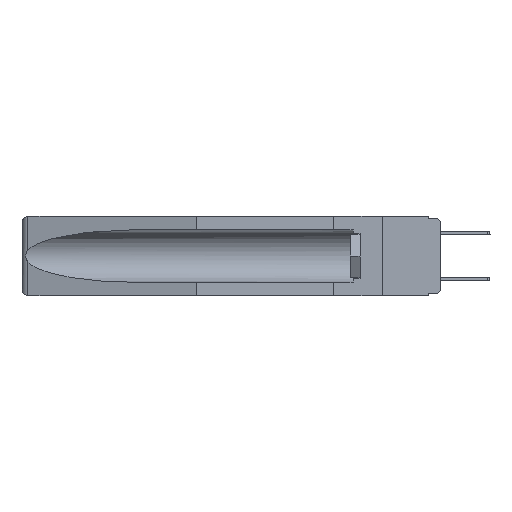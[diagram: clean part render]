
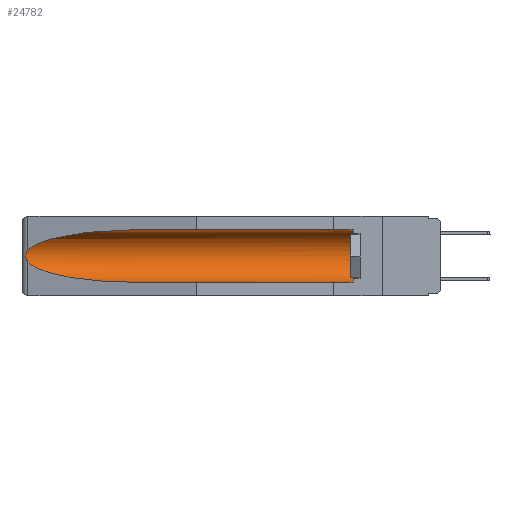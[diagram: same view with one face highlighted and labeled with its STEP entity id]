
A CAD part, left-side view. The second image highlights one B-rep face of the part: STEP entity #24782.
In plain terms, the highlighted cylindrical face has radius 2.857 mm (diameter 5.715 mm), a partial arc.
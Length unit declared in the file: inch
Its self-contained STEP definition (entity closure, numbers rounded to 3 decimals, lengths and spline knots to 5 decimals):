
#196 = DIRECTION ( 'NONE',  ( 0., 0., 1. ) ) ;
#798 = DIRECTION ( 'NONE',  ( 0., 1., 0. ) ) ;
#1414 = CARTESIAN_POINT ( 'NONE',  ( 0.2675, 1.53308, -0.17534 ) ) ;
#1496 = EDGE_CURVE ( 'NONE', #23119, #3552, #24272, .T. ) ;
#1505 = CARTESIAN_POINT ( 'NONE',  ( 0.2673, 1.5327, -0.16383 ) ) ;
#2046 = VERTEX_POINT ( 'NONE', #22098 ) ;
#2772 = CARTESIAN_POINT ( 'NONE',  ( 0.21114, 1.30732, -0.284 ) ) ;
#3189 = CARTESIAN_POINT ( 'NONE',  ( 0.155, 1.07973, -0.059 ) ) ;
#3433 = EDGE_CURVE ( 'NONE', #20549, #22015, #21277, .T. ) ;
#3552 = VERTEX_POINT ( 'NONE', #7488 ) ;
#4908 = ORIENTED_EDGE ( 'NONE', *, *, #1496, .T. ) ;
#5174 = EDGE_CURVE ( 'NONE', #2046, #26042, #6064, .T. ) ;
#5213 = EDGE_CURVE ( 'NONE', #20549, #23119, #16627, .T. ) ;
#6064 = B_SPLINE_CURVE_WITH_KNOTS ( 'NONE', 3,
 ( #16032, #22085, #18098, #1505, #9717, #1414, #24068, #21994, #17839, #19730 ),
 .UNSPECIFIED., .F., .F.,
 ( 4, 2, 2, 2, 4 ),
 ( 0., 0.00029, 0.00058, 0.00087, 0.00117 ),
 .UNSPECIFIED. ) ;
#6332 = EDGE_CURVE ( 'NONE', #26042, #22015, #12840, .T. ) ;
#6385 = CARTESIAN_POINT ( 'NONE',  ( 0.155, 0.126, -0.059 ) ) ;
#7488 = CARTESIAN_POINT ( 'NONE',  ( 0.155, 1.07973, -0.059 ) ) ;
#7738 = DIRECTION ( 'NONE',  ( 0., 0., 1. ) ) ;
#7851 = ORIENTED_EDGE ( 'NONE', *, *, #5174, .T. ) ;
#8418 = EDGE_LOOP ( 'NONE', ( #22985, #7851, #19996, #12005, #13705, #4908 ) ) ;
#8520 = CARTESIAN_POINT ( 'NONE',  ( 0.155, -0.30754, -0.284 ) ) ;
#9717 = CARTESIAN_POINT ( 'NONE',  ( 0.2675, 1.53308, -0.16763 ) ) ;
#10247 = CYLINDRICAL_SURFACE ( 'NONE', #12475, 0.1125 ) ;
#10984 = CARTESIAN_POINT ( 'NONE',  ( 0.25451, 1.48313, -0.24835 ) ) ;
#11436 = AXIS2_PLACEMENT_3D ( 'NONE', #20095, #11538, #7738 ) ;
#11538 = DIRECTION ( 'NONE',  ( 0., -1., 0. ) ) ;
#12005 = ORIENTED_EDGE ( 'NONE', *, *, #3433, .F. ) ;
#12475 = AXIS2_PLACEMENT_3D ( 'NONE', #20961, #12591, #196 ) ;
#12591 = DIRECTION ( 'NONE',  ( 0., 1., 0. ) ) ;
#12840 =( BOUNDED_CURVE ( )  B_SPLINE_CURVE ( 3, ( #14835, #10984, #2772, #13651 ),
 .UNSPECIFIED., .F., .T. ) 
 B_SPLINE_CURVE_WITH_KNOTS ( ( 4, 4 ),
 ( 0.1948, 1.5708 ),
 .UNSPECIFIED. ) 
 CURVE ( )  GEOMETRIC_REPRESENTATION_ITEM ( )  RATIONAL_B_SPLINE_CURVE ( ( 1., 0.848, 0.848, 1. ) ) 
 REPRESENTATION_ITEM ( '' )  );
#13651 = CARTESIAN_POINT ( 'NONE',  ( 0.155, 1.07973, -0.284 ) ) ;
#13705 = ORIENTED_EDGE ( 'NONE', *, *, #5213, .T. ) ;
#14736 = DIRECTION ( 'NONE',  ( 0., 1., 0. ) ) ;
#14835 = CARTESIAN_POINT ( 'NONE',  ( 0.26537, 1.52718, -0.19328 ) ) ;
#16032 = CARTESIAN_POINT ( 'NONE',  ( 0.26537, 1.52718, -0.14972 ) ) ;
#16627 = CIRCLE ( 'NONE', #11436, 0.1125 ) ;
#16700 = EDGE_CURVE ( 'NONE', #3552, #2046, #26759, .T. ) ;
#17839 = CARTESIAN_POINT ( 'NONE',  ( 0.26597, 1.5296, -0.19026 ) ) ;
#18098 = CARTESIAN_POINT ( 'NONE',  ( 0.26654, 1.53092, -0.15636 ) ) ;
#19580 = CARTESIAN_POINT ( 'NONE',  ( 0.25451, 1.48313, -0.09465 ) ) ;
#19730 = CARTESIAN_POINT ( 'NONE',  ( 0.26537, 1.52718, -0.19328 ) ) ;
#19856 = CARTESIAN_POINT ( 'NONE',  ( 0.21114, 1.30732, -0.059 ) ) ;
#19983 = VECTOR ( 'NONE', #14736, 39.37008 ) ;
#19996 = ORIENTED_EDGE ( 'NONE', *, *, #6332, .T. ) ;
#20095 = CARTESIAN_POINT ( 'NONE',  ( 0.155, 0.126, -0.1715 ) ) ;
#20549 = VERTEX_POINT ( 'NONE', #22933 ) ;
#20961 = CARTESIAN_POINT ( 'NONE',  ( 0.155, -0.30754, -0.1715 ) ) ;
#21277 = LINE ( 'NONE', #8520, #19983 ) ;
#21392 = CARTESIAN_POINT ( 'NONE',  ( 0.155, -0.30754, -0.059 ) ) ;
#21994 = CARTESIAN_POINT ( 'NONE',  ( 0.26655, 1.53094, -0.18657 ) ) ;
#22015 = VERTEX_POINT ( 'NONE', #22821 ) ;
#22085 = CARTESIAN_POINT ( 'NONE',  ( 0.26597, 1.52961, -0.15275 ) ) ;
#22098 = CARTESIAN_POINT ( 'NONE',  ( 0.26537, 1.52718, -0.14972 ) ) ;
#22821 = CARTESIAN_POINT ( 'NONE',  ( 0.155, 1.07973, -0.284 ) ) ;
#22933 = CARTESIAN_POINT ( 'NONE',  ( 0.155, 0.126, -0.284 ) ) ;
#22985 = ORIENTED_EDGE ( 'NONE', *, *, #16700, .T. ) ;
#23119 = VERTEX_POINT ( 'NONE', #6385 ) ;
#23618 = VECTOR ( 'NONE', #798, 39.37008 ) ;
#23721 = CARTESIAN_POINT ( 'NONE',  ( 0.26537, 1.52718, -0.14972 ) ) ;
#24068 = CARTESIAN_POINT ( 'NONE',  ( 0.2673, 1.53269, -0.17917 ) ) ;
#24272 = LINE ( 'NONE', #21392, #23618 ) ;
#24782 = ADVANCED_FACE ( 'NONE', ( #25107 ), #10247, .F. ) ;
#25064 = CARTESIAN_POINT ( 'NONE',  ( 0.26537, 1.52718, -0.19328 ) ) ;
#25107 = FACE_OUTER_BOUND ( 'NONE', #8418, .T. ) ;
#26042 = VERTEX_POINT ( 'NONE', #25064 ) ;
#26759 =( BOUNDED_CURVE ( )  B_SPLINE_CURVE ( 3, ( #3189, #19856, #19580, #23721 ),
 .UNSPECIFIED., .F., .T. ) 
 B_SPLINE_CURVE_WITH_KNOTS ( ( 4, 4 ),
 ( 4.71239, 6.08839 ),
 .UNSPECIFIED. ) 
 CURVE ( )  GEOMETRIC_REPRESENTATION_ITEM ( )  RATIONAL_B_SPLINE_CURVE ( ( 1., 0.848, 0.848, 1. ) ) 
 REPRESENTATION_ITEM ( '' )  );
